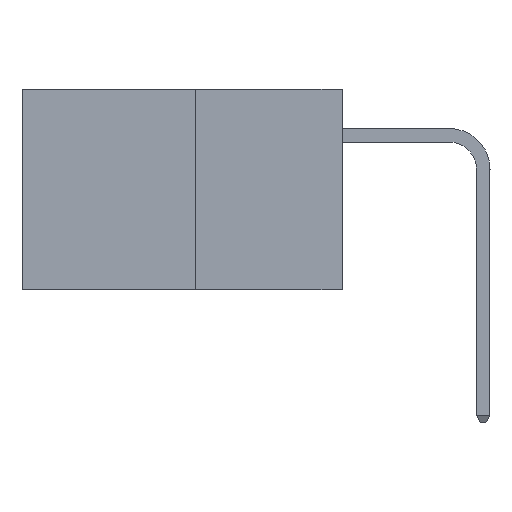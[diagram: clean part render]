
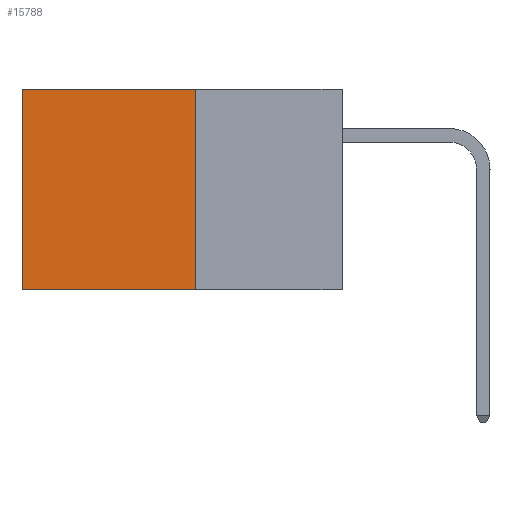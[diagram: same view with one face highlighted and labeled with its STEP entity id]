
A CAD part, left-side view. The second image highlights one B-rep face of the part: STEP entity #15788.
In plain terms, the highlighted planar face has unit normal (-1, 0, 0).
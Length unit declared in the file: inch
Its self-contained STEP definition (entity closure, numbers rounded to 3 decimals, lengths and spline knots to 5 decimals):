
#1333 = VECTOR ( 'NONE', #20099, 39.37008 ) ;
#1714 = EDGE_LOOP ( 'NONE', ( #15123, #9810, #9920, #20795 ) ) ;
#3298 = LINE ( 'NONE', #18127, #15756 ) ;
#4936 = DIRECTION ( 'NONE',  ( 0., 0., -1. ) ) ;
#4996 = EDGE_CURVE ( 'NONE', #14129, #8112, #3298, .T. ) ;
#5915 = VECTOR ( 'NONE', #4936, 39.37008 ) ;
#6039 = DIRECTION ( 'NONE',  ( 1., 0., 0. ) ) ;
#7477 = LINE ( 'NONE', #16074, #16053 ) ;
#7929 = CARTESIAN_POINT ( 'NONE',  ( 0.277, 0.59, 0. ) ) ;
#8112 = VERTEX_POINT ( 'NONE', #18746 ) ;
#8632 = AXIS2_PLACEMENT_3D ( 'NONE', #15730, #6039, #17309 ) ;
#8965 = CARTESIAN_POINT ( 'NONE',  ( 0.277, 0.27, -0.37 ) ) ;
#9810 = ORIENTED_EDGE ( 'NONE', *, *, #4996, .F. ) ;
#9920 = ORIENTED_EDGE ( 'NONE', *, *, #13785, .F. ) ;
#10527 = VERTEX_POINT ( 'NONE', #7929 ) ;
#11388 = CARTESIAN_POINT ( 'NONE',  ( 0.277, 0.27, -0.37 ) ) ;
#12544 = CARTESIAN_POINT ( 'NONE',  ( 0.277, 0.27, 0. ) ) ;
#12760 = EDGE_CURVE ( 'NONE', #10527, #8112, #14315, .T. ) ;
#13785 = EDGE_CURVE ( 'NONE', #19487, #14129, #14522, .T. ) ;
#14084 = PLANE ( 'NONE',  #8632 ) ;
#14129 = VERTEX_POINT ( 'NONE', #8965 ) ;
#14241 = FACE_OUTER_BOUND ( 'NONE', #1714, .T. ) ;
#14315 = LINE ( 'NONE', #18508, #1333 ) ;
#14522 = LINE ( 'NONE', #11388, #5915 ) ;
#15071 = EDGE_CURVE ( 'NONE', #19487, #10527, #7477, .T. ) ;
#15123 = ORIENTED_EDGE ( 'NONE', *, *, #12760, .T. ) ;
#15730 = CARTESIAN_POINT ( 'NONE',  ( 0.277, 0.27, -0.37 ) ) ;
#15756 = VECTOR ( 'NONE', #18110, 39.37008 ) ;
#15788 = ADVANCED_FACE ( 'NONE', ( #14241 ), #14084, .F. ) ;
#16053 = VECTOR ( 'NONE', #17645, 39.37008 ) ;
#16074 = CARTESIAN_POINT ( 'NONE',  ( 0.277, 0.27, 0. ) ) ;
#17309 = DIRECTION ( 'NONE',  ( 0., 0., -1. ) ) ;
#17645 = DIRECTION ( 'NONE',  ( 0., 1., 0. ) ) ;
#18110 = DIRECTION ( 'NONE',  ( 0., 1., 0. ) ) ;
#18127 = CARTESIAN_POINT ( 'NONE',  ( 0.277, 0.27, -0.37 ) ) ;
#18508 = CARTESIAN_POINT ( 'NONE',  ( 0.277, 0.59, -0.37 ) ) ;
#18746 = CARTESIAN_POINT ( 'NONE',  ( 0.277, 0.59, -0.37 ) ) ;
#19487 = VERTEX_POINT ( 'NONE', #12544 ) ;
#20099 = DIRECTION ( 'NONE',  ( 0., 0., -1. ) ) ;
#20795 = ORIENTED_EDGE ( 'NONE', *, *, #15071, .T. ) ;
